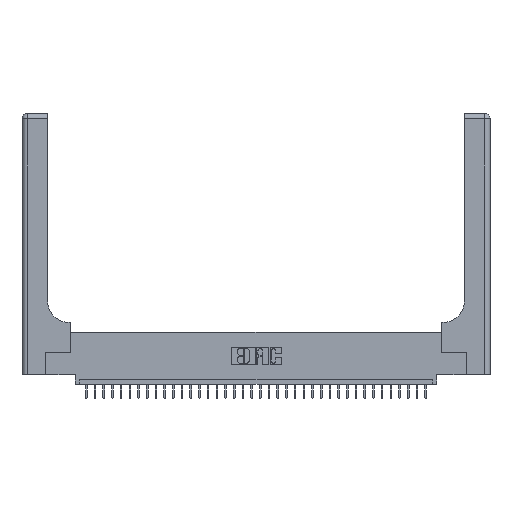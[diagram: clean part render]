
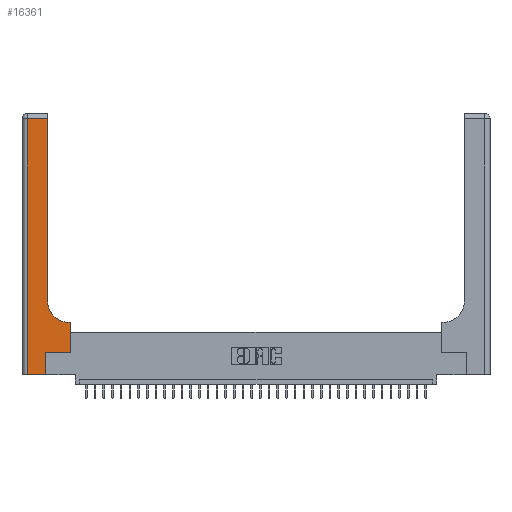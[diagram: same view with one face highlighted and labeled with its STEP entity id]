
A CAD part, top view. The second image highlights one B-rep face of the part: STEP entity #16361.
In plain terms, the highlighted planar face has unit normal (0, 0, 1).
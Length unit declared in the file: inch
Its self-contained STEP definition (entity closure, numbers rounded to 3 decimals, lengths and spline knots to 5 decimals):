
#182 = DIRECTION ( 'NONE',  ( 0., -1., 0. ) ) ;
#433 = CARTESIAN_POINT ( 'NONE',  ( 0.06, 3., 0.37 ) ) ;
#701 = LINE ( 'NONE', #25969, #4184 ) ;
#922 = VERTEX_POINT ( 'NONE', #12096 ) ;
#1241 = ORIENTED_EDGE ( 'NONE', *, *, #31379, .T. ) ;
#2401 = VERTEX_POINT ( 'NONE', #29427 ) ;
#2463 = LINE ( 'NONE', #433, #28350 ) ;
#2510 = CARTESIAN_POINT ( 'NONE',  ( 0., 3., 0.37 ) ) ;
#2562 = VECTOR ( 'NONE', #23461, 39.37008 ) ;
#2968 = CARTESIAN_POINT ( 'NONE',  ( 0.5585, 0.25, 0.37 ) ) ;
#3074 = ORIENTED_EDGE ( 'NONE', *, *, #13397, .T. ) ;
#3125 = VECTOR ( 'NONE', #16229, 39.37008 ) ;
#3541 = DIRECTION ( 'NONE',  ( 0., 0., -1. ) ) ;
#3722 = ORIENTED_EDGE ( 'NONE', *, *, #25487, .T. ) ;
#3788 = DIRECTION ( 'NONE',  ( 1., 0., 0. ) ) ;
#4184 = VECTOR ( 'NONE', #12129, 39.37008 ) ;
#4930 = VERTEX_POINT ( 'NONE', #5858 ) ;
#5359 = DIRECTION ( 'NONE',  ( 0., 0., -1. ) ) ;
#5492 = DIRECTION ( 'NONE',  ( 0., 1., 0. ) ) ;
#5726 = CARTESIAN_POINT ( 'NONE',  ( 0.06, 2.94, 0.37 ) ) ;
#5821 = VERTEX_POINT ( 'NONE', #13799 ) ;
#5858 = CARTESIAN_POINT ( 'NONE',  ( 0.269, 0.25, 0.37 ) ) ;
#6941 = CARTESIAN_POINT ( 'NONE',  ( 0.5415, 0.6, 0.37 ) ) ;
#7271 = FACE_OUTER_BOUND ( 'NONE', #16710, .T. ) ;
#9279 = VECTOR ( 'NONE', #13331, 39.37008 ) ;
#9454 = EDGE_CURVE ( 'NONE', #5821, #28244, #13585, .T. ) ;
#11671 = EDGE_CURVE ( 'NONE', #16378, #27904, #13048, .T. ) ;
#11913 = EDGE_CURVE ( 'NONE', #4930, #2401, #17369, .T. ) ;
#12096 = CARTESIAN_POINT ( 'NONE',  ( 0.2915, 0.85, 0.37 ) ) ;
#12129 = DIRECTION ( 'NONE',  ( -1., 0., 0. ) ) ;
#13048 = LINE ( 'NONE', #32737, #3125 ) ;
#13331 = DIRECTION ( 'NONE',  ( 1., 0., 0. ) ) ;
#13397 = EDGE_CURVE ( 'NONE', #28244, #4930, #21385, .T. ) ;
#13562 = CARTESIAN_POINT ( 'NONE',  ( 0., 0., 0.37 ) ) ;
#13585 = LINE ( 'NONE', #13562, #9279 ) ;
#13799 = CARTESIAN_POINT ( 'NONE',  ( 0.06, 0., 0.37 ) ) ;
#14221 = ORIENTED_EDGE ( 'NONE', *, *, #26520, .T. ) ;
#14584 = ORIENTED_EDGE ( 'NONE', *, *, #9454, .T. ) ;
#15249 = CARTESIAN_POINT ( 'NONE',  ( 0.269, 0., 0.37 ) ) ;
#16229 = DIRECTION ( 'NONE',  ( -1., 0., 0. ) ) ;
#16361 = ADVANCED_FACE ( 'NONE', ( #7271 ), #35667, .F. ) ;
#16378 = VERTEX_POINT ( 'NONE', #24835 ) ;
#16710 = EDGE_LOOP ( 'NONE', ( #1241, #35096, #3722, #14584, #3074, #27734, #33510, #30595, #14221 ) ) ;
#17041 = CARTESIAN_POINT ( 'NONE',  ( 0.5415, 0.85, 0.37 ) ) ;
#17369 = LINE ( 'NONE', #33469, #27715 ) ;
#19369 = LINE ( 'NONE', #20672, #2562 ) ;
#19871 = DIRECTION ( 'NONE',  ( 1., 0., 0. ) ) ;
#19948 = CARTESIAN_POINT ( 'NONE',  ( 0.2915, 2.94, 0.37 ) ) ;
#20117 = DIRECTION ( 'NONE',  ( 0., 1., 0. ) ) ;
#20293 = VECTOR ( 'NONE', #5492, 39.37008 ) ;
#20672 = CARTESIAN_POINT ( 'NONE',  ( 0.2915, 3., 0.37 ) ) ;
#21385 = LINE ( 'NONE', #25813, #22206 ) ;
#21846 = VERTEX_POINT ( 'NONE', #19948 ) ;
#22206 = VECTOR ( 'NONE', #20117, 39.37008 ) ;
#22946 = LINE ( 'NONE', #2968, #20293 ) ;
#23216 = CIRCLE ( 'NONE', #35368, 0.25 ) ;
#23461 = DIRECTION ( 'NONE',  ( 0., 1., 0. ) ) ;
#23852 = EDGE_CURVE ( 'NONE', #2401, #16378, #22946, .T. ) ;
#24835 = CARTESIAN_POINT ( 'NONE',  ( 0.5585, 0.6, 0.37 ) ) ;
#25487 = EDGE_CURVE ( 'NONE', #34108, #5821, #2463, .T. ) ;
#25813 = CARTESIAN_POINT ( 'NONE',  ( 0.269, 0., 0.37 ) ) ;
#25969 = CARTESIAN_POINT ( 'NONE',  ( 0., 2.94, 0.37 ) ) ;
#26520 = EDGE_CURVE ( 'NONE', #27904, #922, #23216, .T. ) ;
#27715 = VECTOR ( 'NONE', #19871, 39.37008 ) ;
#27734 = ORIENTED_EDGE ( 'NONE', *, *, #11913, .T. ) ;
#27904 = VERTEX_POINT ( 'NONE', #6941 ) ;
#28244 = VERTEX_POINT ( 'NONE', #15249 ) ;
#28350 = VECTOR ( 'NONE', #182, 39.37008 ) ;
#29427 = CARTESIAN_POINT ( 'NONE',  ( 0.5585, 0.25, 0.37 ) ) ;
#30595 = ORIENTED_EDGE ( 'NONE', *, *, #11671, .T. ) ;
#31379 = EDGE_CURVE ( 'NONE', #922, #21846, #19369, .T. ) ;
#32620 = EDGE_CURVE ( 'NONE', #21846, #34108, #701, .T. ) ;
#32737 = CARTESIAN_POINT ( 'NONE',  ( 0.2915, 0.6, 0.37 ) ) ;
#32988 = DIRECTION ( 'NONE',  ( -1., 0., 0. ) ) ;
#33469 = CARTESIAN_POINT ( 'NONE',  ( 0.269, 0.25, 0.37 ) ) ;
#33510 = ORIENTED_EDGE ( 'NONE', *, *, #23852, .T. ) ;
#34108 = VERTEX_POINT ( 'NONE', #5726 ) ;
#35096 = ORIENTED_EDGE ( 'NONE', *, *, #32620, .T. ) ;
#35159 = AXIS2_PLACEMENT_3D ( 'NONE', #2510, #5359, #32988 ) ;
#35368 = AXIS2_PLACEMENT_3D ( 'NONE', #17041, #3541, #3788 ) ;
#35667 = PLANE ( 'NONE',  #35159 ) ;
